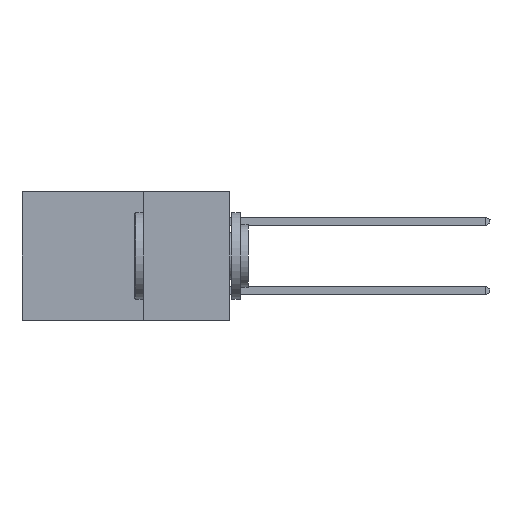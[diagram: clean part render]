
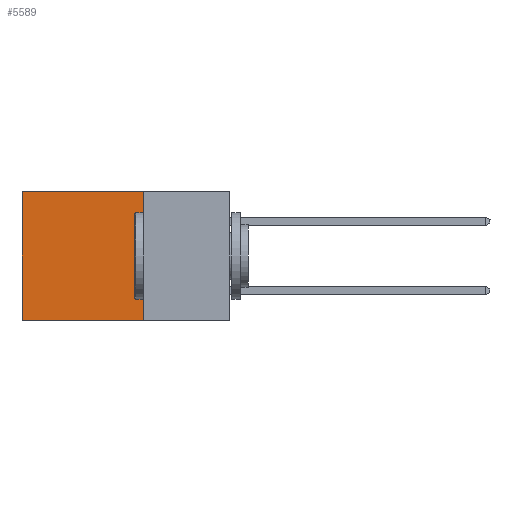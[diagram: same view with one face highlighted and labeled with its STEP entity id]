
A CAD part, left-side view. The second image highlights one B-rep face of the part: STEP entity #5589.
In plain terms, the highlighted planar face has unit normal (-1, 0, 0).
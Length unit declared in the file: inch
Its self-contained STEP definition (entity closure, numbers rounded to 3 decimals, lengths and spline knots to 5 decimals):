
#211 = FACE_OUTER_BOUND ( 'NONE', #1598, .T. ) ;
#279 = CARTESIAN_POINT ( 'NONE',  ( 0.298, 0.25, 0. ) ) ;
#656 = VECTOR ( 'NONE', #15876, 39.37008 ) ;
#874 = VERTEX_POINT ( 'NONE', #15026 ) ;
#1598 = EDGE_LOOP ( 'NONE', ( #8296, #17031, #3193, #4254 ) ) ;
#2618 = DIRECTION ( 'NONE',  ( 0., 1., 0. ) ) ;
#3104 = CARTESIAN_POINT ( 'NONE',  ( 0.298, 0.25, 0. ) ) ;
#3160 = DIRECTION ( 'NONE',  ( 0., 0., -1. ) ) ;
#3193 = ORIENTED_EDGE ( 'NONE', *, *, #6069, .F. ) ;
#4254 = ORIENTED_EDGE ( 'NONE', *, *, #18506, .T. ) ;
#5147 = LINE ( 'NONE', #11036, #656 ) ;
#5589 = ADVANCED_FACE ( 'NONE', ( #211 ), #7695, .F. ) ;
#6069 = EDGE_CURVE ( 'NONE', #16328, #874, #19007, .T. ) ;
#7109 = EDGE_CURVE ( 'NONE', #874, #12770, #11643, .T. ) ;
#7646 = DIRECTION ( 'NONE',  ( 1., 0., 0. ) ) ;
#7695 = PLANE ( 'NONE',  #14681 ) ;
#8133 = VECTOR ( 'NONE', #17630, 39.37008 ) ;
#8296 = ORIENTED_EDGE ( 'NONE', *, *, #8523, .T. ) ;
#8523 = EDGE_CURVE ( 'NONE', #18095, #12770, #5147, .T. ) ;
#11036 = CARTESIAN_POINT ( 'NONE',  ( 0.298, 0.6, 0. ) ) ;
#11643 = LINE ( 'NONE', #13901, #20217 ) ;
#12374 = LINE ( 'NONE', #3104, #8133 ) ;
#12770 = VERTEX_POINT ( 'NONE', #17044 ) ;
#13901 = CARTESIAN_POINT ( 'NONE',  ( 0.298, 0.25, -0.37 ) ) ;
#14563 = DIRECTION ( 'NONE',  ( 0., 0., -1. ) ) ;
#14681 = AXIS2_PLACEMENT_3D ( 'NONE', #19311, #7646, #3160 ) ;
#14709 = VECTOR ( 'NONE', #14563, 39.37008 ) ;
#15026 = CARTESIAN_POINT ( 'NONE',  ( 0.298, 0.25, -0.37 ) ) ;
#15269 = CARTESIAN_POINT ( 'NONE',  ( 0.298, 0.25, 0. ) ) ;
#15876 = DIRECTION ( 'NONE',  ( 0., 0., -1. ) ) ;
#16328 = VERTEX_POINT ( 'NONE', #15269 ) ;
#17031 = ORIENTED_EDGE ( 'NONE', *, *, #7109, .F. ) ;
#17044 = CARTESIAN_POINT ( 'NONE',  ( 0.298, 0.6, -0.37 ) ) ;
#17630 = DIRECTION ( 'NONE',  ( 0., 1., 0. ) ) ;
#18095 = VERTEX_POINT ( 'NONE', #18195 ) ;
#18195 = CARTESIAN_POINT ( 'NONE',  ( 0.298, 0.6, 0. ) ) ;
#18506 = EDGE_CURVE ( 'NONE', #16328, #18095, #12374, .T. ) ;
#19007 = LINE ( 'NONE', #279, #14709 ) ;
#19311 = CARTESIAN_POINT ( 'NONE',  ( 0.298, 0.25, 0. ) ) ;
#20217 = VECTOR ( 'NONE', #2618, 39.37008 ) ;
